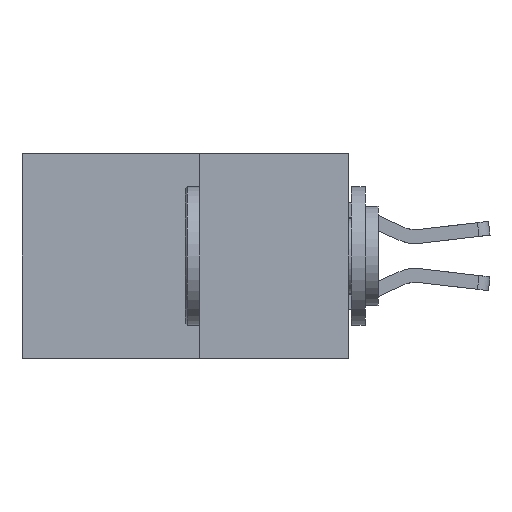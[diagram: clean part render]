
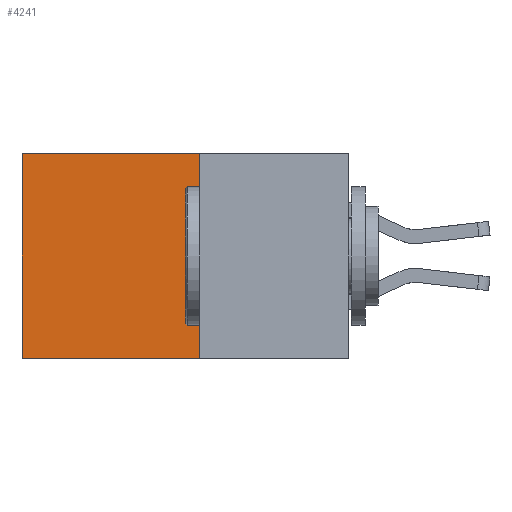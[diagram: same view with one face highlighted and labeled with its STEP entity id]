
A CAD part, left-side view. The second image highlights one B-rep face of the part: STEP entity #4241.
In plain terms, the highlighted planar face has unit normal (-1, 0, 0).
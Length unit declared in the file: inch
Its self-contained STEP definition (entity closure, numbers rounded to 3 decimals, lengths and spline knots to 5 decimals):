
#330 = ORIENTED_EDGE ( 'NONE', *, *, #2068, .F. ) ;
#406 = VERTEX_POINT ( 'NONE', #8972 ) ;
#503 = VERTEX_POINT ( 'NONE', #5572 ) ;
#583 = VECTOR ( 'NONE', #5202, 39.37008 ) ;
#735 = EDGE_CURVE ( 'NONE', #8677, #406, #10701, .T. ) ;
#1436 = EDGE_CURVE ( 'NONE', #8677, #5309, #11376, .T. ) ;
#1487 = VECTOR ( 'NONE', #10605, 39.37008 ) ;
#2068 = EDGE_CURVE ( 'NONE', #5309, #503, #10912, .T. ) ;
#2241 = CARTESIAN_POINT ( 'NONE',  ( 0.277, 0.27, -0.37 ) ) ;
#2911 = DIRECTION ( 'NONE',  ( 0., 0., -1. ) ) ;
#2998 = DIRECTION ( 'NONE',  ( 1., 0., 0. ) ) ;
#3017 = PLANE ( 'NONE',  #7564 ) ;
#3115 = CARTESIAN_POINT ( 'NONE',  ( 0.277, 0.27, -0.37 ) ) ;
#3466 = CARTESIAN_POINT ( 'NONE',  ( 0.277, 0.27, 0. ) ) ;
#4241 = ADVANCED_FACE ( 'NONE', ( #8903 ), #3017, .F. ) ;
#4583 = ORIENTED_EDGE ( 'NONE', *, *, #7232, .T. ) ;
#5202 = DIRECTION ( 'NONE',  ( 0., 1., 0. ) ) ;
#5309 = VERTEX_POINT ( 'NONE', #7159 ) ;
#5572 = CARTESIAN_POINT ( 'NONE',  ( 0.277, 0.59, -0.37 ) ) ;
#7159 = CARTESIAN_POINT ( 'NONE',  ( 0.277, 0.27, -0.37 ) ) ;
#7232 = EDGE_CURVE ( 'NONE', #406, #503, #9252, .T. ) ;
#7564 = AXIS2_PLACEMENT_3D ( 'NONE', #3115, #2998, #2911 ) ;
#7705 = ORIENTED_EDGE ( 'NONE', *, *, #1436, .F. ) ;
#7847 = DIRECTION ( 'NONE',  ( 0., 0., -1. ) ) ;
#8114 = CARTESIAN_POINT ( 'NONE',  ( 0.277, 0.27, 0. ) ) ;
#8442 = ORIENTED_EDGE ( 'NONE', *, *, #735, .T. ) ;
#8511 = EDGE_LOOP ( 'NONE', ( #4583, #330, #7705, #8442 ) ) ;
#8677 = VERTEX_POINT ( 'NONE', #3466 ) ;
#8903 = FACE_OUTER_BOUND ( 'NONE', #8511, .T. ) ;
#8972 = CARTESIAN_POINT ( 'NONE',  ( 0.277, 0.59, 0. ) ) ;
#9037 = DIRECTION ( 'NONE',  ( 0., 1., 0. ) ) ;
#9252 = LINE ( 'NONE', #9720, #1487 ) ;
#9720 = CARTESIAN_POINT ( 'NONE',  ( 0.277, 0.59, -0.37 ) ) ;
#10417 = VECTOR ( 'NONE', #9037, 39.37008 ) ;
#10605 = DIRECTION ( 'NONE',  ( 0., 0., -1. ) ) ;
#10701 = LINE ( 'NONE', #8114, #10417 ) ;
#10912 = LINE ( 'NONE', #11731, #583 ) ;
#11101 = VECTOR ( 'NONE', #7847, 39.37008 ) ;
#11376 = LINE ( 'NONE', #2241, #11101 ) ;
#11731 = CARTESIAN_POINT ( 'NONE',  ( 0.277, 0.27, -0.37 ) ) ;
